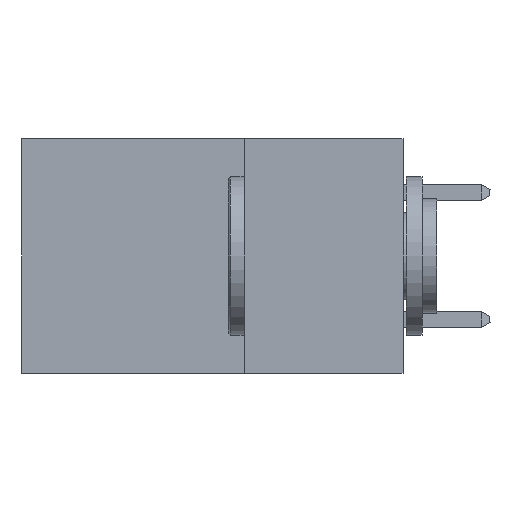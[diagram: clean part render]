
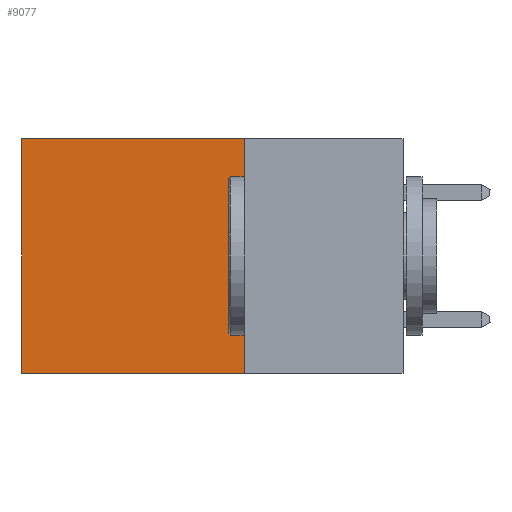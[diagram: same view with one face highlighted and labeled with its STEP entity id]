
A CAD part, left-side view. The second image highlights one B-rep face of the part: STEP entity #9077.
In plain terms, the highlighted planar face has unit normal (-1, 0, 0).
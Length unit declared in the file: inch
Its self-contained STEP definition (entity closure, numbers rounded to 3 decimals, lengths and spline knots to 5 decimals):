
#1033 = CARTESIAN_POINT ( 'NONE',  ( 0.2875, 0.25, -0.37 ) ) ;
#1111 = CARTESIAN_POINT ( 'NONE',  ( 0.2875, 0.6, 0. ) ) ;
#1222 = DIRECTION ( 'NONE',  ( 0., 0., -1. ) ) ;
#1589 = DIRECTION ( 'NONE',  ( 0., 0., -1. ) ) ;
#1595 = EDGE_LOOP ( 'NONE', ( #2253, #8982, #11993, #12478 ) ) ;
#2005 = LINE ( 'NONE', #1111, #7760 ) ;
#2088 = CARTESIAN_POINT ( 'NONE',  ( 0.2875, 0.25, 0. ) ) ;
#2186 = CARTESIAN_POINT ( 'NONE',  ( 0.2875, 0.25, 0. ) ) ;
#2253 = ORIENTED_EDGE ( 'NONE', *, *, #3743, .T. ) ;
#3678 = DIRECTION ( 'NONE',  ( 0., 1., 0. ) ) ;
#3743 = EDGE_CURVE ( 'NONE', #9698, #5729, #2005, .T. ) ;
#3846 = EDGE_CURVE ( 'NONE', #6081, #9698, #9998, .T. ) ;
#5729 = VERTEX_POINT ( 'NONE', #6589 ) ;
#6081 = VERTEX_POINT ( 'NONE', #2088 ) ;
#6215 = PLANE ( 'NONE',  #7190 ) ;
#6589 = CARTESIAN_POINT ( 'NONE',  ( 0.2875, 0.6, -0.37 ) ) ;
#7190 = AXIS2_PLACEMENT_3D ( 'NONE', #16667, #18074, #1589 ) ;
#7232 = CARTESIAN_POINT ( 'NONE',  ( 0.2875, 0.25, 0. ) ) ;
#7694 = FACE_OUTER_BOUND ( 'NONE', #1595, .T. ) ;
#7760 = VECTOR ( 'NONE', #17710, 39.37008 ) ;
#7864 = EDGE_CURVE ( 'NONE', #6081, #17501, #11046, .T. ) ;
#8339 = VECTOR ( 'NONE', #3678, 39.37008 ) ;
#8982 = ORIENTED_EDGE ( 'NONE', *, *, #17054, .F. ) ;
#9077 = ADVANCED_FACE ( 'NONE', ( #7694 ), #6215, .F. ) ;
#9170 = CARTESIAN_POINT ( 'NONE',  ( 0.2875, 0.25, -0.37 ) ) ;
#9593 = CARTESIAN_POINT ( 'NONE',  ( 0.2875, 0.6, 0. ) ) ;
#9698 = VERTEX_POINT ( 'NONE', #9593 ) ;
#9998 = LINE ( 'NONE', #2186, #8339 ) ;
#11046 = LINE ( 'NONE', #7232, #14541 ) ;
#11993 = ORIENTED_EDGE ( 'NONE', *, *, #7864, .F. ) ;
#12478 = ORIENTED_EDGE ( 'NONE', *, *, #3846, .T. ) ;
#12731 = DIRECTION ( 'NONE',  ( 0., 1., 0. ) ) ;
#14498 = LINE ( 'NONE', #1033, #16360 ) ;
#14541 = VECTOR ( 'NONE', #1222, 39.37008 ) ;
#16360 = VECTOR ( 'NONE', #12731, 39.37008 ) ;
#16667 = CARTESIAN_POINT ( 'NONE',  ( 0.2875, 0.25, 0. ) ) ;
#17054 = EDGE_CURVE ( 'NONE', #17501, #5729, #14498, .T. ) ;
#17501 = VERTEX_POINT ( 'NONE', #9170 ) ;
#17710 = DIRECTION ( 'NONE',  ( 0., 0., -1. ) ) ;
#18074 = DIRECTION ( 'NONE',  ( 1., 0., 0. ) ) ;
